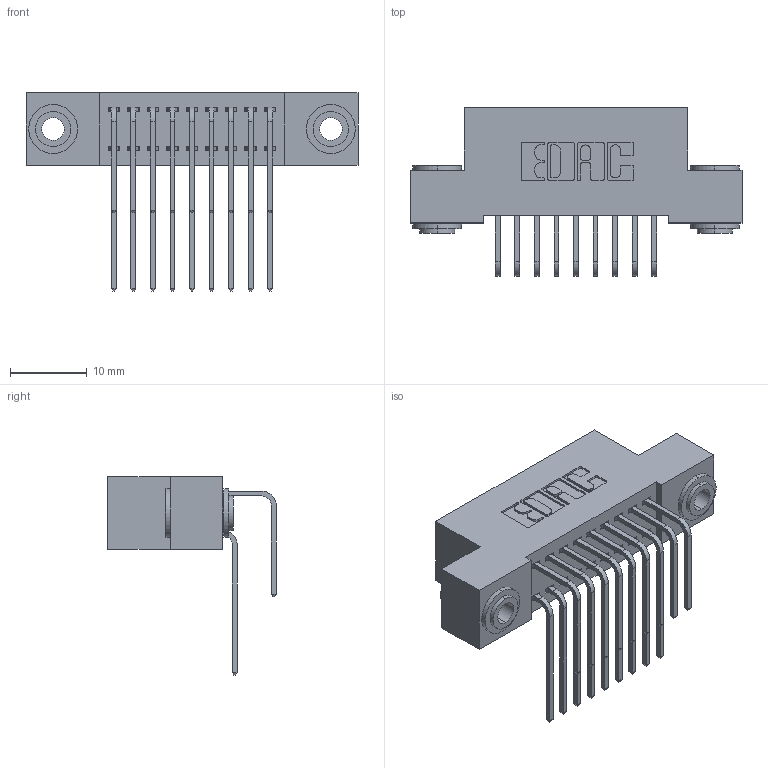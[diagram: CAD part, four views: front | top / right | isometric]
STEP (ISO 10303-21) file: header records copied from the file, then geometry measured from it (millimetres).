
FILE_DESCRIPTION (( 'STEP AP203' ), '1' );
FILE_NAME ('342-018-558-203.STEP', '2018-08-10T21:50:22', ( '' ), ( '' ), 'SwSTEP 2.0', 'SolidWorks 2016', '' );
FILE_SCHEMA (( 'CONFIG_CONTROL_DESIGN' ));
Length unit declared in the file: inch
Products named in the file (5): 342 Part_.156 TH; 345-292-001_558 559 Tail - 1; 345-292-001_558 Tail - 2; 342-250-002_345-250-002-102; 342-018-558-203
Assembly tree (21 placements, depth 2):
  342-018-558-203
    342 Part_.156 TH
    345-292-001_558 559 Tail - 1  x9
    345-292-001_558 Tail - 2  x9
    342-250-002_345-250-002-102  x2
Bounding box: 43.18 x 21.91 x 25.78 mm (x, y, z)
Volume: 3850.2 mm3; surface area: 6137.8 mm2
Topology: 21 solids, 21 shells, 1120 faces, 3273 edges, 2154 vertices
Faces by surface type: plane 760, cylinder 352, cone 8
Entity records: 12360 total; most frequent: CARTESIAN_POINT 2112, ORIENTED_EDGE 1990, DIRECTION 1877, EDGE_CURVE 995, LINE 803, VECTOR 803, VERTEX_POINT 658, AXIS2_PLACEMENT_3D 537
